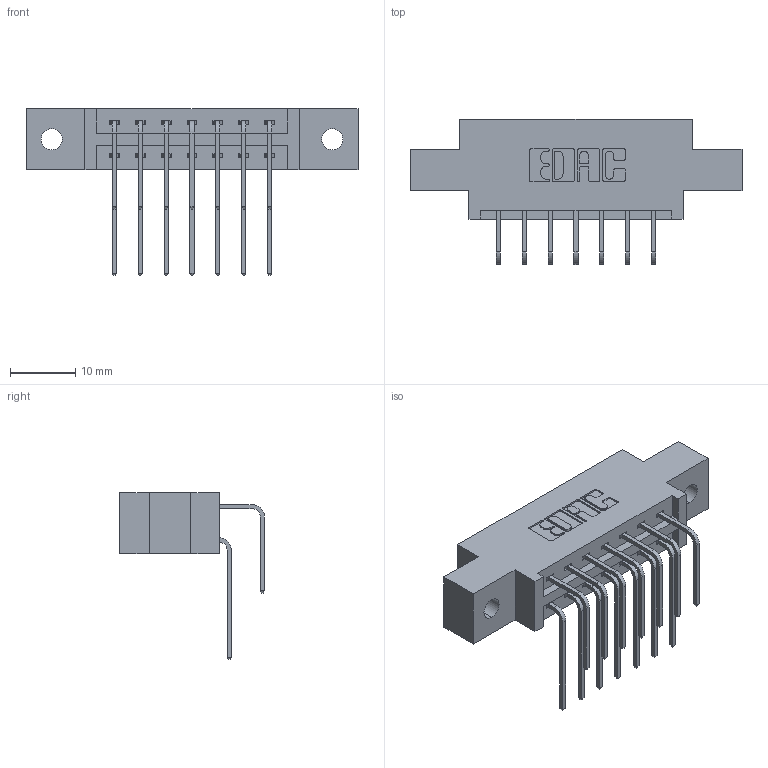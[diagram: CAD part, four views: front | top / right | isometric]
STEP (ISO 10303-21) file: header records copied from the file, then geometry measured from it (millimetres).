
FILE_DESCRIPTION (( 'STEP AP203' ), '1' );
FILE_NAME ('387-014-558-802.STEP', '2018-09-11T06:12:16', ( '' ), ( '' ), 'SwSTEP 2.0', 'SolidWorks 2016', '' );
FILE_SCHEMA (( 'CONFIG_CONTROL_DESIGN' ));
Length unit declared in the file: inch
Products named in the file (4): 337 Part_0.170 Offset - 0.128 Dia; 345-292-001_558 559 Tail - 1; 345-292-001_558 Tail - 2; 387-014-558-802
Assembly tree (15 placements, depth 2):
  387-014-558-802
    337 Part_0.170 Offset - 0.128 Dia
    345-292-001_558 559 Tail - 1  x7
    345-292-001_558 Tail - 2  x7
Bounding box: 50.75 x 22.17 x 25.53 mm (x, y, z)
Volume: 4809 mm3; surface area: 5337.3 mm2
Topology: 15 solids, 15 shells, 902 faces, 2661 edges, 1754 vertices
Faces by surface type: plane 634, cylinder 268
Entity records: 11873 total; most frequent: CARTESIAN_POINT 2077, ORIENTED_EDGE 1962, DIRECTION 1813, EDGE_CURVE 981, LINE 813, VECTOR 813, VERTEX_POINT 650, AXIS2_PLACEMENT_3D 500
